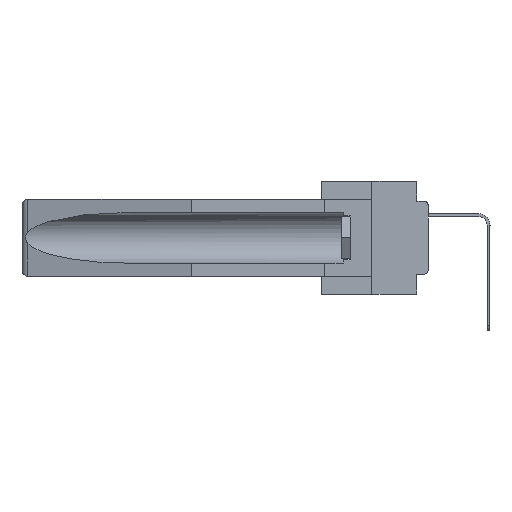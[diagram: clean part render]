
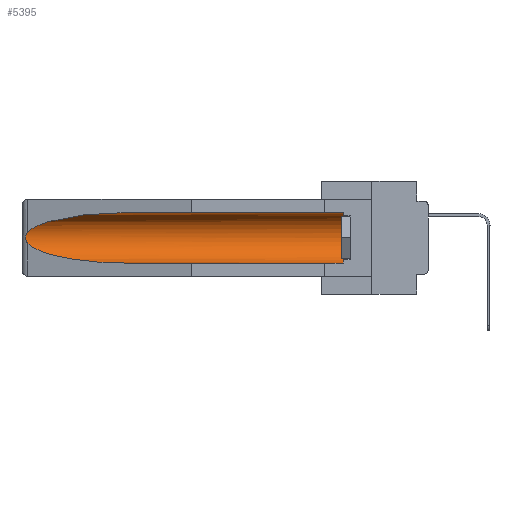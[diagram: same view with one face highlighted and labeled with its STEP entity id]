
A CAD part, left-side view. The second image highlights one B-rep face of the part: STEP entity #5395.
In plain terms, the highlighted cylindrical face has radius 2.857 mm (diameter 5.715 mm), a partial arc.
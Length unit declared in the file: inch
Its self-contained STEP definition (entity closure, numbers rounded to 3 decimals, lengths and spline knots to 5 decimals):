
#306 = ORIENTED_EDGE ( 'NONE', *, *, #19360, .T. ) ;
#517 = CARTESIAN_POINT ( 'NONE',  ( 0.155, 0.126, -0.059 ) ) ;
#1122 = CARTESIAN_POINT ( 'NONE',  ( 0.26537, 1.52718, -0.19328 ) ) ;
#2383 = ORIENTED_EDGE ( 'NONE', *, *, #29366, .T. ) ;
#2402 = DIRECTION ( 'NONE',  ( 0., 0., 1. ) ) ;
#2778 = CARTESIAN_POINT ( 'NONE',  ( 0.26537, 1.52718, -0.14972 ) ) ;
#3613 = CARTESIAN_POINT ( 'NONE',  ( 0.26537, 1.52718, -0.19328 ) ) ;
#3787 = EDGE_CURVE ( 'NONE', #10814, #10282, #22106, .T. ) ;
#5318 = CARTESIAN_POINT ( 'NONE',  ( 0.26537, 1.52718, -0.14972 ) ) ;
#5367 = CARTESIAN_POINT ( 'NONE',  ( 0.155, -0.30754, -0.1715 ) ) ;
#5395 = ADVANCED_FACE ( 'NONE', ( #24535 ), #13761, .F. ) ;
#5460 = DIRECTION ( 'NONE',  ( 0., 1., 0. ) ) ;
#5771 = ORIENTED_EDGE ( 'NONE', *, *, #12964, .T. ) ;
#5847 = VECTOR ( 'NONE', #16554, 39.37008 ) ;
#6354 = CIRCLE ( 'NONE', #21013, 0.1125 ) ;
#6367 = EDGE_CURVE ( 'NONE', #9100, #14262, #14643, .T. ) ;
#6741 =( BOUNDED_CURVE ( )  B_SPLINE_CURVE ( 3, ( #19244, #12333, #23659, #5318 ),
 .UNSPECIFIED., .F., .T. ) 
 B_SPLINE_CURVE_WITH_KNOTS ( ( 4, 4 ),
 ( 4.71239, 6.08839 ),
 .UNSPECIFIED. ) 
 CURVE ( )  GEOMETRIC_REPRESENTATION_ITEM ( )  RATIONAL_B_SPLINE_CURVE ( ( 1., 0.848, 0.848, 1. ) ) 
 REPRESENTATION_ITEM ( '' )  );
#7357 = CARTESIAN_POINT ( 'NONE',  ( 0.155, -0.30754, -0.059 ) ) ;
#7758 = CARTESIAN_POINT ( 'NONE',  ( 0.26655, 1.53094, -0.18657 ) ) ;
#8169 = CARTESIAN_POINT ( 'NONE',  ( 0.26654, 1.53092, -0.15636 ) ) ;
#9100 = VERTEX_POINT ( 'NONE', #2778 ) ;
#9387 = CARTESIAN_POINT ( 'NONE',  ( 0.155, 1.07973, -0.059 ) ) ;
#10262 = CARTESIAN_POINT ( 'NONE',  ( 0.2675, 1.53308, -0.17534 ) ) ;
#10282 = VERTEX_POINT ( 'NONE', #16424 ) ;
#10814 = VERTEX_POINT ( 'NONE', #20607 ) ;
#11088 = AXIS2_PLACEMENT_3D ( 'NONE', #5367, #5460, #23705 ) ;
#11768 = VERTEX_POINT ( 'NONE', #517 ) ;
#12333 = CARTESIAN_POINT ( 'NONE',  ( 0.21114, 1.30732, -0.059 ) ) ;
#12372 = CARTESIAN_POINT ( 'NONE',  ( 0.2675, 1.53308, -0.16763 ) ) ;
#12964 = EDGE_CURVE ( 'NONE', #14262, #10282, #26436, .T. ) ;
#13444 = ORIENTED_EDGE ( 'NONE', *, *, #6367, .T. ) ;
#13761 = CYLINDRICAL_SURFACE ( 'NONE', #11088, 0.1125 ) ;
#14130 = CARTESIAN_POINT ( 'NONE',  ( 0.155, 0.126, -0.1715 ) ) ;
#14228 = EDGE_CURVE ( 'NONE', #21189, #9100, #6741, .T. ) ;
#14262 = VERTEX_POINT ( 'NONE', #16731 ) ;
#14643 = B_SPLINE_CURVE_WITH_KNOTS ( 'NONE', 3,
 ( #24100, #21786, #8169, #16853, #12372, #10262, #21480, #7758, #23787, #1122 ),
 .UNSPECIFIED., .F., .F.,
 ( 4, 2, 2, 2, 4 ),
 ( 0., 0.00029, 0.00058, 0.00087, 0.00117 ),
 .UNSPECIFIED. ) ;
#16113 = DIRECTION ( 'NONE',  ( 0., -1., 0. ) ) ;
#16424 = CARTESIAN_POINT ( 'NONE',  ( 0.155, 1.07973, -0.284 ) ) ;
#16554 = DIRECTION ( 'NONE',  ( 0., 1., 0. ) ) ;
#16731 = CARTESIAN_POINT ( 'NONE',  ( 0.26537, 1.52718, -0.19328 ) ) ;
#16853 = CARTESIAN_POINT ( 'NONE',  ( 0.2673, 1.5327, -0.16383 ) ) ;
#16920 = CARTESIAN_POINT ( 'NONE',  ( 0.155, 1.07973, -0.284 ) ) ;
#17385 = DIRECTION ( 'NONE',  ( 0., 1., 0. ) ) ;
#18943 = EDGE_LOOP ( 'NONE', ( #25650, #13444, #5771, #28975, #306, #2383 ) ) ;
#19244 = CARTESIAN_POINT ( 'NONE',  ( 0.155, 1.07973, -0.059 ) ) ;
#19360 = EDGE_CURVE ( 'NONE', #10814, #11768, #6354, .T. ) ;
#19658 = CARTESIAN_POINT ( 'NONE',  ( 0.25451, 1.48313, -0.24835 ) ) ;
#20607 = CARTESIAN_POINT ( 'NONE',  ( 0.155, 0.126, -0.284 ) ) ;
#21013 = AXIS2_PLACEMENT_3D ( 'NONE', #14130, #16113, #2402 ) ;
#21189 = VERTEX_POINT ( 'NONE', #9387 ) ;
#21480 = CARTESIAN_POINT ( 'NONE',  ( 0.2673, 1.53269, -0.17917 ) ) ;
#21786 = CARTESIAN_POINT ( 'NONE',  ( 0.26597, 1.52961, -0.15275 ) ) ;
#22106 = LINE ( 'NONE', #23800, #24271 ) ;
#23659 = CARTESIAN_POINT ( 'NONE',  ( 0.25451, 1.48313, -0.09465 ) ) ;
#23705 = DIRECTION ( 'NONE',  ( 0., 0., 1. ) ) ;
#23787 = CARTESIAN_POINT ( 'NONE',  ( 0.26597, 1.5296, -0.19026 ) ) ;
#23800 = CARTESIAN_POINT ( 'NONE',  ( 0.155, -0.30754, -0.284 ) ) ;
#24100 = CARTESIAN_POINT ( 'NONE',  ( 0.26537, 1.52718, -0.14972 ) ) ;
#24148 = LINE ( 'NONE', #7357, #5847 ) ;
#24271 = VECTOR ( 'NONE', #17385, 39.37008 ) ;
#24535 = FACE_OUTER_BOUND ( 'NONE', #18943, .T. ) ;
#25650 = ORIENTED_EDGE ( 'NONE', *, *, #14228, .T. ) ;
#26436 =( BOUNDED_CURVE ( )  B_SPLINE_CURVE ( 3, ( #3613, #19658, #28620, #16920 ),
 .UNSPECIFIED., .F., .T. ) 
 B_SPLINE_CURVE_WITH_KNOTS ( ( 4, 4 ),
 ( 0.1948, 1.5708 ),
 .UNSPECIFIED. ) 
 CURVE ( )  GEOMETRIC_REPRESENTATION_ITEM ( )  RATIONAL_B_SPLINE_CURVE ( ( 1., 0.848, 0.848, 1. ) ) 
 REPRESENTATION_ITEM ( '' )  );
#28620 = CARTESIAN_POINT ( 'NONE',  ( 0.21114, 1.30732, -0.284 ) ) ;
#28975 = ORIENTED_EDGE ( 'NONE', *, *, #3787, .F. ) ;
#29366 = EDGE_CURVE ( 'NONE', #11768, #21189, #24148, .T. ) ;
